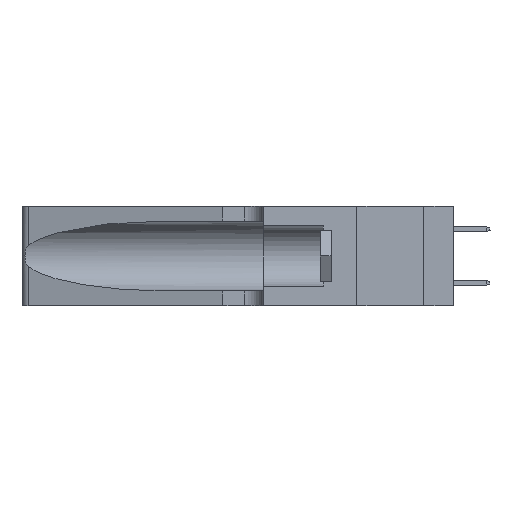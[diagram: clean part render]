
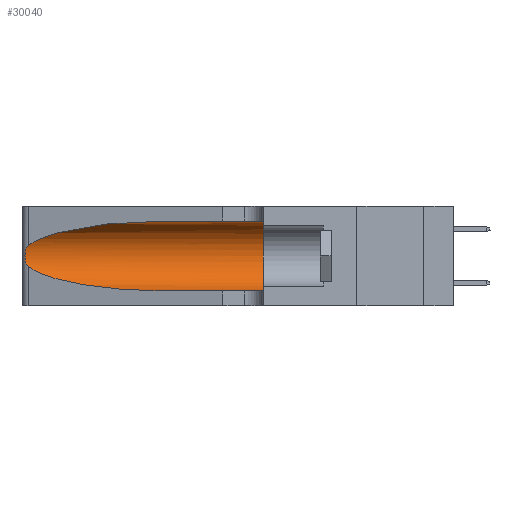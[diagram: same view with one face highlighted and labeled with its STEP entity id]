
A CAD part, left-side view. The second image highlights one B-rep face of the part: STEP entity #30040.
In plain terms, the highlighted cylindrical face has radius 3.308 mm (diameter 6.617 mm), a partial arc.
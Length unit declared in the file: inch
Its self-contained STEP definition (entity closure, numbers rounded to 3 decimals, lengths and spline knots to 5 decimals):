
#73 = CARTESIAN_POINT ( 'NONE',  ( 0.26075, 1.23896, 0.19203 ) ) ;
#989 = VERTEX_POINT ( 'NONE', #43771 ) ;
#1395 = DIRECTION ( 'NONE',  ( 0., -1., 0. ) ) ;
#2601 = VERTEX_POINT ( 'NONE', #18268 ) ;
#3146 = VECTOR ( 'NONE', #8176, 39.37008 ) ;
#3158 = CARTESIAN_POINT ( 'NONE',  ( 0.1305, 0.35, 0.185 ) ) ;
#3321 = EDGE_LOOP ( 'NONE', ( #5544, #5827, #10943, #36051, #24079, #41274 ) ) ;
#4062 =( BOUNDED_CURVE ( )  B_SPLINE_CURVE ( 3, ( #18199, #21448, #7558, #17982 ),
 .UNSPECIFIED., .F., .F. ) 
 B_SPLINE_CURVE_WITH_KNOTS ( ( 4, 4 ),
 ( 3.44316, 4.71239 ),
 .UNSPECIFIED. ) 
 CURVE ( )  GEOMETRIC_REPRESENTATION_ITEM ( )  RATIONAL_B_SPLINE_CURVE ( ( 1., 0.87, 0.87, 1. ) ) 
 REPRESENTATION_ITEM ( '' )  );
#5037 = LINE ( 'NONE', #25652, #43310 ) ;
#5544 = ORIENTED_EDGE ( 'NONE', *, *, #6642, .T. ) ;
#5827 = ORIENTED_EDGE ( 'NONE', *, *, #39122, .T. ) ;
#5908 = CARTESIAN_POINT ( 'NONE',  ( 0.1305, 0.35, 0.05475 ) ) ;
#6642 = EDGE_CURVE ( 'NONE', #989, #42548, #29750, .T. ) ;
#7558 = CARTESIAN_POINT ( 'NONE',  ( 0.18966, 0.96281, 0.05475 ) ) ;
#7639 = CARTESIAN_POINT ( 'NONE',  ( 0.25487, 1.22718, 0.22369 ) ) ;
#8176 = DIRECTION ( 'NONE',  ( 0., -1., 0. ) ) ;
#8345 = CARTESIAN_POINT ( 'NONE',  ( 0.26018, 1.23835, 0.19895 ) ) ;
#8574 = CARTESIAN_POINT ( 'NONE',  ( 0.26075, 1.23896, 0.178 ) ) ;
#10566 = DIRECTION ( 'NONE',  ( 0., 0., 1. ) ) ;
#10745 = CARTESIAN_POINT ( 'NONE',  ( 0.25856, 1.23593, 0.16098 ) ) ;
#10943 = ORIENTED_EDGE ( 'NONE', *, *, #32100, .T. ) ;
#12068 = CARTESIAN_POINT ( 'NONE',  ( 0.25787, 1.23484, 0.2124 ) ) ;
#15304 = CARTESIAN_POINT ( 'NONE',  ( 0.25555, 1.22994, 0.2215 ) ) ;
#15533 = FACE_OUTER_BOUND ( 'NONE', #3321, .T. ) ;
#15998 = CYLINDRICAL_SURFACE ( 'NONE', #31741, 0.13025 ) ;
#16556 = CARTESIAN_POINT ( 'NONE',  ( 0.25487, 1.22718, 0.14631 ) ) ;
#17457 = CIRCLE ( 'NONE', #36635, 0.13025 ) ;
#17982 = CARTESIAN_POINT ( 'NONE',  ( 0.1305, 0.72297, 0.05475 ) ) ;
#18199 = CARTESIAN_POINT ( 'NONE',  ( 0.25487, 1.22718, 0.14631 ) ) ;
#18268 = CARTESIAN_POINT ( 'NONE',  ( 0.1305, 0.35, 0.31525 ) ) ;
#18334 = CARTESIAN_POINT ( 'NONE',  ( 0.2373, 1.15595, 0.28018 ) ) ;
#18575 = VERTEX_POINT ( 'NONE', #26341 ) ;
#18599 = CARTESIAN_POINT ( 'NONE',  ( 0.1305, 1.61858, 0.31525 ) ) ;
#18612 = B_SPLINE_CURVE_WITH_KNOTS ( 'NONE', 3,
 ( #25960, #15304, #32863, #12068, #21155, #8345, #73, #8574, #43761, #10745, #39799, #29866, #26183, #40271 ),
 .UNSPECIFIED., .F., .F.,
 ( 4, 2, 2, 2, 2, 2, 4 ),
 ( 0., 0.00027, 0.00053, 0.00107, 0.0016, 0.00187, 0.00214 ),
 .UNSPECIFIED. ) ;
#18819 = EDGE_CURVE ( 'NONE', #2601, #31018, #17457, .T. ) ;
#18984 = CARTESIAN_POINT ( 'NONE',  ( 0.1305, 1.61858, 0.185 ) ) ;
#21155 = CARTESIAN_POINT ( 'NONE',  ( 0.25854, 1.2359, 0.20912 ) ) ;
#21448 = CARTESIAN_POINT ( 'NONE',  ( 0.2373, 1.15595, 0.08982 ) ) ;
#21805 = CARTESIAN_POINT ( 'NONE',  ( 0.18966, 0.96281, 0.31525 ) ) ;
#22921 = DIRECTION ( 'NONE',  ( 0., 0., -1. ) ) ;
#24079 = ORIENTED_EDGE ( 'NONE', *, *, #18819, .F. ) ;
#24895 = DIRECTION ( 'NONE',  ( 0., 1., 0. ) ) ;
#25652 = CARTESIAN_POINT ( 'NONE',  ( 0.1305, 1.61858, 0.05475 ) ) ;
#25960 = CARTESIAN_POINT ( 'NONE',  ( 0.25487, 1.22718, 0.22369 ) ) ;
#26183 = CARTESIAN_POINT ( 'NONE',  ( 0.25555, 1.22993, 0.14849 ) ) ;
#26341 = CARTESIAN_POINT ( 'NONE',  ( 0.1305, 0.72297, 0.05475 ) ) ;
#29750 =( BOUNDED_CURVE ( )  B_SPLINE_CURVE ( 3, ( #39375, #21805, #18334, #32435 ),
 .UNSPECIFIED., .F., .F. ) 
 B_SPLINE_CURVE_WITH_KNOTS ( ( 4, 4 ),
 ( 1.5708, 2.84003 ),
 .UNSPECIFIED. ) 
 CURVE ( )  GEOMETRIC_REPRESENTATION_ITEM ( )  RATIONAL_B_SPLINE_CURVE ( ( 1., 0.87, 0.87, 1. ) ) 
 REPRESENTATION_ITEM ( '' )  );
#29779 = VERTEX_POINT ( 'NONE', #16556 ) ;
#29866 = CARTESIAN_POINT ( 'NONE',  ( 0.25639, 1.23186, 0.15144 ) ) ;
#30040 = ADVANCED_FACE ( 'NONE', ( #15533 ), #15998, .F. ) ;
#31018 = VERTEX_POINT ( 'NONE', #5908 ) ;
#31741 = AXIS2_PLACEMENT_3D ( 'NONE', #18984, #1395, #22921 ) ;
#32100 = EDGE_CURVE ( 'NONE', #29779, #18575, #4062, .T. ) ;
#32435 = CARTESIAN_POINT ( 'NONE',  ( 0.25487, 1.22718, 0.22369 ) ) ;
#32461 = LINE ( 'NONE', #18599, #3146 ) ;
#32863 = CARTESIAN_POINT ( 'NONE',  ( 0.25639, 1.23184, 0.21858 ) ) ;
#33262 = DIRECTION ( 'NONE',  ( 0., -1., 0. ) ) ;
#34516 = EDGE_CURVE ( 'NONE', #989, #2601, #32461, .T. ) ;
#36051 = ORIENTED_EDGE ( 'NONE', *, *, #45591, .T. ) ;
#36635 = AXIS2_PLACEMENT_3D ( 'NONE', #3158, #24895, #10566 ) ;
#39122 = EDGE_CURVE ( 'NONE', #42548, #29779, #18612, .T. ) ;
#39375 = CARTESIAN_POINT ( 'NONE',  ( 0.1305, 0.72297, 0.31525 ) ) ;
#39799 = CARTESIAN_POINT ( 'NONE',  ( 0.25789, 1.23486, 0.15765 ) ) ;
#40271 = CARTESIAN_POINT ( 'NONE',  ( 0.25487, 1.22718, 0.14631 ) ) ;
#41274 = ORIENTED_EDGE ( 'NONE', *, *, #34516, .F. ) ;
#42548 = VERTEX_POINT ( 'NONE', #7639 ) ;
#43310 = VECTOR ( 'NONE', #33262, 39.37008 ) ;
#43761 = CARTESIAN_POINT ( 'NONE',  ( 0.26017, 1.23833, 0.17102 ) ) ;
#43771 = CARTESIAN_POINT ( 'NONE',  ( 0.1305, 0.72297, 0.31525 ) ) ;
#45591 = EDGE_CURVE ( 'NONE', #18575, #31018, #5037, .T. ) ;
